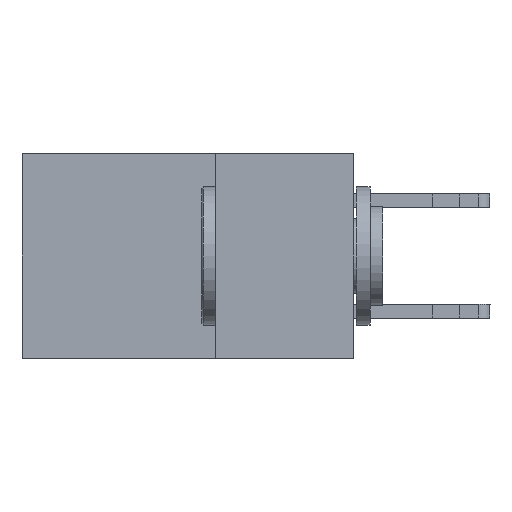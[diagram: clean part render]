
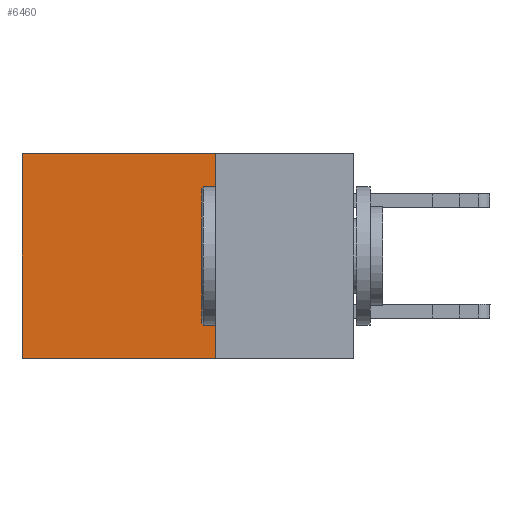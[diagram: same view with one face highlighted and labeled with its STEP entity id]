
A CAD part, left-side view. The second image highlights one B-rep face of the part: STEP entity #6460.
In plain terms, the highlighted planar face has unit normal (-1, 0, 0).
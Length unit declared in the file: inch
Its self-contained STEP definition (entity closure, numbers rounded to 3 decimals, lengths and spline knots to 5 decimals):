
#137 = VERTEX_POINT ( 'NONE', #13021 ) ;
#867 = CARTESIAN_POINT ( 'NONE',  ( 0.2875, 0.25, 0. ) ) ;
#2417 = DIRECTION ( 'NONE',  ( 0., 1., 0. ) ) ;
#2701 = DIRECTION ( 'NONE',  ( 0., 1., 0. ) ) ;
#3358 = PLANE ( 'NONE',  #12964 ) ;
#3492 = EDGE_CURVE ( 'NONE', #8801, #137, #17685, .T. ) ;
#4357 = CARTESIAN_POINT ( 'NONE',  ( 0.2875, 0.6, 0. ) ) ;
#4416 = DIRECTION ( 'NONE',  ( 0., 0., -1. ) ) ;
#4537 = DIRECTION ( 'NONE',  ( 1., 0., 0. ) ) ;
#5568 = CARTESIAN_POINT ( 'NONE',  ( 0.2875, 0.25, -0.37 ) ) ;
#5868 = CARTESIAN_POINT ( 'NONE',  ( 0.2875, 0.25, 0. ) ) ;
#6018 = FACE_OUTER_BOUND ( 'NONE', #6839, .T. ) ;
#6410 = VECTOR ( 'NONE', #4416, 39.37008 ) ;
#6460 = ADVANCED_FACE ( 'NONE', ( #6018 ), #3358, .F. ) ;
#6839 = EDGE_LOOP ( 'NONE', ( #6917, #9779, #9318, #13322 ) ) ;
#6917 = ORIENTED_EDGE ( 'NONE', *, *, #3492, .T. ) ;
#8370 = LINE ( 'NONE', #5568, #10093 ) ;
#8801 = VERTEX_POINT ( 'NONE', #13744 ) ;
#8903 = LINE ( 'NONE', #19227, #6410 ) ;
#9112 = CARTESIAN_POINT ( 'NONE',  ( 0.2875, 0.25, 0. ) ) ;
#9318 = ORIENTED_EDGE ( 'NONE', *, *, #15510, .F. ) ;
#9779 = ORIENTED_EDGE ( 'NONE', *, *, #17827, .F. ) ;
#10093 = VECTOR ( 'NONE', #2417, 39.37008 ) ;
#12964 = AXIS2_PLACEMENT_3D ( 'NONE', #9112, #4537, #13611 ) ;
#13021 = CARTESIAN_POINT ( 'NONE',  ( 0.2875, 0.6, -0.37 ) ) ;
#13041 = DIRECTION ( 'NONE',  ( 0., 0., -1. ) ) ;
#13322 = ORIENTED_EDGE ( 'NONE', *, *, #16864, .T. ) ;
#13611 = DIRECTION ( 'NONE',  ( 0., 0., -1. ) ) ;
#13744 = CARTESIAN_POINT ( 'NONE',  ( 0.2875, 0.6, 0. ) ) ;
#13861 = CARTESIAN_POINT ( 'NONE',  ( 0.2875, 0.25, -0.37 ) ) ;
#13866 = VECTOR ( 'NONE', #13041, 39.37008 ) ;
#14036 = VERTEX_POINT ( 'NONE', #5868 ) ;
#15510 = EDGE_CURVE ( 'NONE', #14036, #17666, #8903, .T. ) ;
#16072 = LINE ( 'NONE', #867, #18122 ) ;
#16864 = EDGE_CURVE ( 'NONE', #14036, #8801, #16072, .T. ) ;
#17666 = VERTEX_POINT ( 'NONE', #13861 ) ;
#17685 = LINE ( 'NONE', #4357, #13866 ) ;
#17827 = EDGE_CURVE ( 'NONE', #17666, #137, #8370, .T. ) ;
#18122 = VECTOR ( 'NONE', #2701, 39.37008 ) ;
#19227 = CARTESIAN_POINT ( 'NONE',  ( 0.2875, 0.25, 0. ) ) ;
